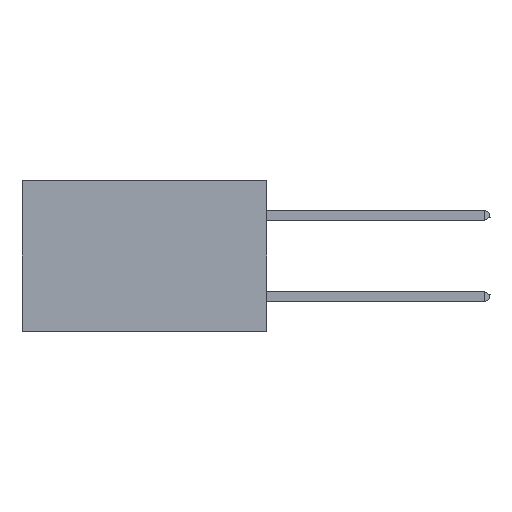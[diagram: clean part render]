
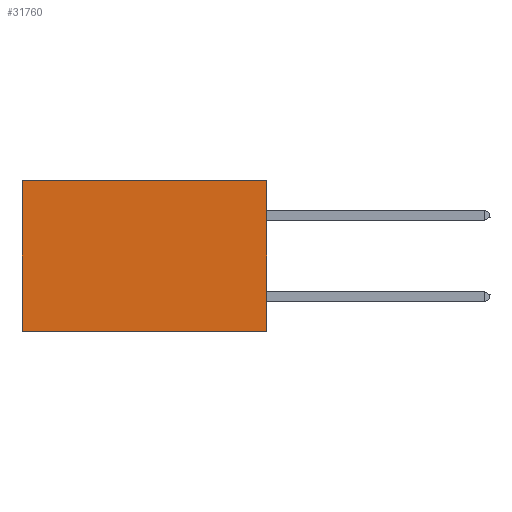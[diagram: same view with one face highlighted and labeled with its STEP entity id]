
A CAD part, left-side view. The second image highlights one B-rep face of the part: STEP entity #31760.
In plain terms, the highlighted planar face has unit normal (-1, 0, 0).
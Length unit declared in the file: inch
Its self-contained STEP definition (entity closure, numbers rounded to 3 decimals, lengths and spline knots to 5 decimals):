
#395 = ORIENTED_EDGE ( 'NONE', *, *, #21682, .F. ) ;
#1068 = VECTOR ( 'NONE', #4526, 39.37008 ) ;
#1323 = FACE_OUTER_BOUND ( 'NONE', #20909, .T. ) ;
#1338 = ORIENTED_EDGE ( 'NONE', *, *, #33314, .T. ) ;
#1759 = CARTESIAN_POINT ( 'NONE',  ( 0.2875, 0., 0. ) ) ;
#2030 = LINE ( 'NONE', #7985, #29320 ) ;
#2629 = ORIENTED_EDGE ( 'NONE', *, *, #30875, .T. ) ;
#3016 = LINE ( 'NONE', #8957, #33274 ) ;
#3735 = PLANE ( 'NONE',  #28824 ) ;
#4526 = DIRECTION ( 'NONE',  ( 0., 0., -1. ) ) ;
#5481 = CARTESIAN_POINT ( 'NONE',  ( 0.2875, 0., 0. ) ) ;
#5724 = DIRECTION ( 'NONE',  ( 0., 1., 0. ) ) ;
#6914 = VERTEX_POINT ( 'NONE', #5481 ) ;
#6950 = LINE ( 'NONE', #27570, #10711 ) ;
#7985 = CARTESIAN_POINT ( 'NONE',  ( 0.2875, 0., 0. ) ) ;
#8957 = CARTESIAN_POINT ( 'NONE',  ( 0.2875, 0., -0.37 ) ) ;
#9333 = VERTEX_POINT ( 'NONE', #12038 ) ;
#10711 = VECTOR ( 'NONE', #32724, 39.37008 ) ;
#12038 = CARTESIAN_POINT ( 'NONE',  ( 0.2875, 0., -0.37 ) ) ;
#20909 = EDGE_LOOP ( 'NONE', ( #2629, #395, #31494, #1338 ) ) ;
#21682 = EDGE_CURVE ( 'NONE', #9333, #27170, #3016, .T. ) ;
#22766 = CARTESIAN_POINT ( 'NONE',  ( 0.2875, 0., 0. ) ) ;
#25486 = DIRECTION ( 'NONE',  ( 1., 0., 0. ) ) ;
#25513 = EDGE_CURVE ( 'NONE', #6914, #9333, #31331, .T. ) ;
#27170 = VERTEX_POINT ( 'NONE', #34622 ) ;
#27570 = CARTESIAN_POINT ( 'NONE',  ( 0.2875, 0.6, 0. ) ) ;
#28824 = AXIS2_PLACEMENT_3D ( 'NONE', #22766, #25486, #30987 ) ;
#29320 = VECTOR ( 'NONE', #5724, 39.37008 ) ;
#30875 = EDGE_CURVE ( 'NONE', #33193, #27170, #6950, .T. ) ;
#30987 = DIRECTION ( 'NONE',  ( 0., 0., -1. ) ) ;
#31331 = LINE ( 'NONE', #1759, #1068 ) ;
#31352 = CARTESIAN_POINT ( 'NONE',  ( 0.2875, 0.6, 0. ) ) ;
#31494 = ORIENTED_EDGE ( 'NONE', *, *, #25513, .F. ) ;
#31760 = ADVANCED_FACE ( 'NONE', ( #1323 ), #3735, .F. ) ;
#32724 = DIRECTION ( 'NONE',  ( 0., 0., -1. ) ) ;
#33193 = VERTEX_POINT ( 'NONE', #31352 ) ;
#33274 = VECTOR ( 'NONE', #33409, 39.37008 ) ;
#33314 = EDGE_CURVE ( 'NONE', #6914, #33193, #2030, .T. ) ;
#33409 = DIRECTION ( 'NONE',  ( 0., 1., 0. ) ) ;
#34622 = CARTESIAN_POINT ( 'NONE',  ( 0.2875, 0.6, -0.37 ) ) ;
